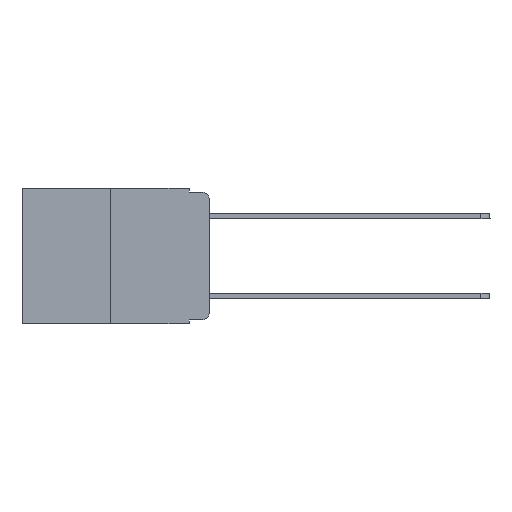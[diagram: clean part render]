
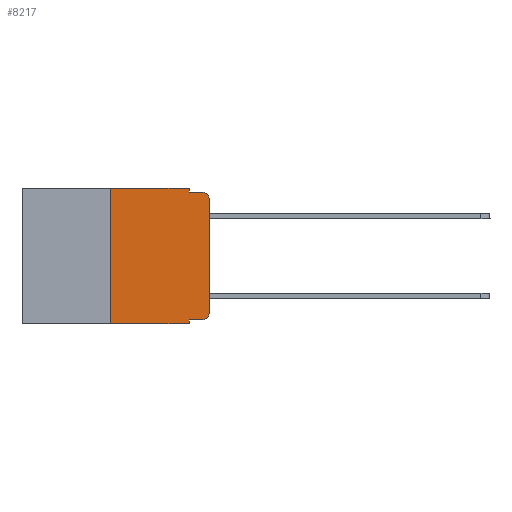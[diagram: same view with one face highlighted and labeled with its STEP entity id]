
A CAD part, left-side view. The second image highlights one B-rep face of the part: STEP entity #8217.
In plain terms, the highlighted planar face has unit normal (-1, 0, 0).
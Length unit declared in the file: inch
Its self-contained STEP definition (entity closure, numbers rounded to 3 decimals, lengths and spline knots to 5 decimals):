
#103 = CARTESIAN_POINT ( 'NONE',  ( 0., 0.473, -0.343 ) ) ;
#1280 = ORIENTED_EDGE ( 'NONE', *, *, #12384, .F. ) ;
#1489 = ORIENTED_EDGE ( 'NONE', *, *, #16381, .F. ) ;
#1766 = ORIENTED_EDGE ( 'NONE', *, *, #16132, .T. ) ;
#2002 = LINE ( 'NONE', #7423, #2789 ) ;
#2565 = VERTEX_POINT ( 'NONE', #9223 ) ;
#2576 = DIRECTION ( 'NONE',  ( 0., 0., -1. ) ) ;
#2789 = VECTOR ( 'NONE', #16298, 39.37008 ) ;
#3077 = ORIENTED_EDGE ( 'NONE', *, *, #19242, .F. ) ;
#3103 = VECTOR ( 'NONE', #5128, 39.37008 ) ;
#4131 = VERTEX_POINT ( 'NONE', #14587 ) ;
#4317 = EDGE_CURVE ( 'NONE', #4131, #9299, #13771, .T. ) ;
#4612 = CARTESIAN_POINT ( 'NONE',  ( 0., 0.473, 0. ) ) ;
#4680 = VERTEX_POINT ( 'NONE', #11216 ) ;
#4949 = CARTESIAN_POINT ( 'NONE',  ( 0., 0.051, 0. ) ) ;
#4962 = ORIENTED_EDGE ( 'NONE', *, *, #18019, .F. ) ;
#5003 = LINE ( 'NONE', #5231, #19151 ) ;
#5128 = DIRECTION ( 'NONE',  ( 0., 0., 1. ) ) ;
#5231 = CARTESIAN_POINT ( 'NONE',  ( 0., 0.051, -0.333 ) ) ;
#6435 = EDGE_CURVE ( 'NONE', #2565, #4680, #17169, .T. ) ;
#6721 = AXIS2_PLACEMENT_3D ( 'NONE', #15763, #7001, #22454 ) ;
#6932 = AXIS2_PLACEMENT_3D ( 'NONE', #4612, #10032, #8307 ) ;
#7001 = DIRECTION ( 'NONE',  ( -1., 0., 0. ) ) ;
#7327 = LINE ( 'NONE', #16428, #18209 ) ;
#7423 = CARTESIAN_POINT ( 'NONE',  ( 0., 0.473, 0. ) ) ;
#8217 = ADVANCED_FACE ( 'NONE', ( #20410 ), #13500, .F. ) ;
#8307 = DIRECTION ( 'NONE',  ( 0., 0., -1. ) ) ;
#8365 = EDGE_CURVE ( 'NONE', #18562, #4680, #8644, .T. ) ;
#8644 = LINE ( 'NONE', #103, #10241 ) ;
#8735 = VERTEX_POINT ( 'NONE', #11399 ) ;
#9223 = CARTESIAN_POINT ( 'NONE',  ( 0., 0.051, -0.333 ) ) ;
#9255 = CARTESIAN_POINT ( 'NONE',  ( 0., 0.02, -0.333 ) ) ;
#9299 = VERTEX_POINT ( 'NONE', #16907 ) ;
#9807 = DIRECTION ( 'NONE',  ( -1., 0., 0. ) ) ;
#10032 = DIRECTION ( 'NONE',  ( 1., 0., 0. ) ) ;
#10241 = VECTOR ( 'NONE', #22711, 39.37008 ) ;
#10306 = DIRECTION ( 'NONE',  ( 0., -1., 0. ) ) ;
#10320 = VECTOR ( 'NONE', #2576, 39.37008 ) ;
#10908 = ORIENTED_EDGE ( 'NONE', *, *, #6435, .F. ) ;
#11216 = CARTESIAN_POINT ( 'NONE',  ( 0., 0.051, -0.343 ) ) ;
#11399 = CARTESIAN_POINT ( 'NONE',  ( 0., 0.051, 0. ) ) ;
#11650 = VERTEX_POINT ( 'NONE', #12645 ) ;
#12145 = EDGE_CURVE ( 'NONE', #2565, #18097, #5003, .T. ) ;
#12384 = EDGE_CURVE ( 'NONE', #8735, #14027, #12956, .T. ) ;
#12518 = DIRECTION ( 'NONE',  ( 0., -1., 0. ) ) ;
#12645 = CARTESIAN_POINT ( 'NONE',  ( 0., 0.02, -0.01 ) ) ;
#12745 = CIRCLE ( 'NONE', #14586, 0.02 ) ;
#12956 = LINE ( 'NONE', #19975, #10320 ) ;
#13125 = CARTESIAN_POINT ( 'NONE',  ( 0., 0.25, 0. ) ) ;
#13315 = ORIENTED_EDGE ( 'NONE', *, *, #19942, .T. ) ;
#13500 = PLANE ( 'NONE',  #6932 ) ;
#13504 = DIRECTION ( 'NONE',  ( 0., 0., -1. ) ) ;
#13771 = LINE ( 'NONE', #20693, #17950 ) ;
#13895 = CARTESIAN_POINT ( 'NONE',  ( 0., 0.25, 0. ) ) ;
#13927 = VECTOR ( 'NONE', #20525, 39.37008 ) ;
#14027 = VERTEX_POINT ( 'NONE', #16375 ) ;
#14586 = AXIS2_PLACEMENT_3D ( 'NONE', #22254, #9807, #13504 ) ;
#14587 = CARTESIAN_POINT ( 'NONE',  ( 0., 0., -0.313 ) ) ;
#15724 = DIRECTION ( 'NONE',  ( 0., 0., 1. ) ) ;
#15729 = LINE ( 'NONE', #13895, #3103 ) ;
#15763 = CARTESIAN_POINT ( 'NONE',  ( 0., 0.02, -0.313 ) ) ;
#16132 = EDGE_CURVE ( 'NONE', #18097, #4131, #20709, .T. ) ;
#16298 = DIRECTION ( 'NONE',  ( 0., -1., 0. ) ) ;
#16375 = CARTESIAN_POINT ( 'NONE',  ( 0., 0.051, -0.01 ) ) ;
#16381 = EDGE_CURVE ( 'NONE', #14027, #11650, #7327, .T. ) ;
#16428 = CARTESIAN_POINT ( 'NONE',  ( 0., 0.051, -0.01 ) ) ;
#16793 = ORIENTED_EDGE ( 'NONE', *, *, #4317, .T. ) ;
#16907 = CARTESIAN_POINT ( 'NONE',  ( 0., 0., -0.03 ) ) ;
#16982 = ORIENTED_EDGE ( 'NONE', *, *, #8365, .T. ) ;
#17169 = LINE ( 'NONE', #4949, #13927 ) ;
#17266 = VERTEX_POINT ( 'NONE', #13125 ) ;
#17950 = VECTOR ( 'NONE', #15724, 39.37008 ) ;
#18019 = EDGE_CURVE ( 'NONE', #18562, #17266, #15729, .T. ) ;
#18097 = VERTEX_POINT ( 'NONE', #9255 ) ;
#18209 = VECTOR ( 'NONE', #12518, 39.37008 ) ;
#18562 = VERTEX_POINT ( 'NONE', #18878 ) ;
#18878 = CARTESIAN_POINT ( 'NONE',  ( 0., 0.25, -0.343 ) ) ;
#19151 = VECTOR ( 'NONE', #10306, 39.37008 ) ;
#19242 = EDGE_CURVE ( 'NONE', #17266, #8735, #2002, .T. ) ;
#19729 = ORIENTED_EDGE ( 'NONE', *, *, #12145, .T. ) ;
#19942 = EDGE_CURVE ( 'NONE', #9299, #11650, #12745, .T. ) ;
#19975 = CARTESIAN_POINT ( 'NONE',  ( 0., 0.051, 0. ) ) ;
#20410 = FACE_OUTER_BOUND ( 'NONE', #22456, .T. ) ;
#20525 = DIRECTION ( 'NONE',  ( 0., 0., -1. ) ) ;
#20693 = CARTESIAN_POINT ( 'NONE',  ( 0., 0., 0. ) ) ;
#20709 = CIRCLE ( 'NONE', #6721, 0.02 ) ;
#22254 = CARTESIAN_POINT ( 'NONE',  ( 0., 0.02, -0.03 ) ) ;
#22454 = DIRECTION ( 'NONE',  ( 0., 0., -1. ) ) ;
#22456 = EDGE_LOOP ( 'NONE', ( #16793, #13315, #1489, #1280, #3077, #4962, #16982, #10908, #19729, #1766 ) ) ;
#22711 = DIRECTION ( 'NONE',  ( 0., -1., 0. ) ) ;
